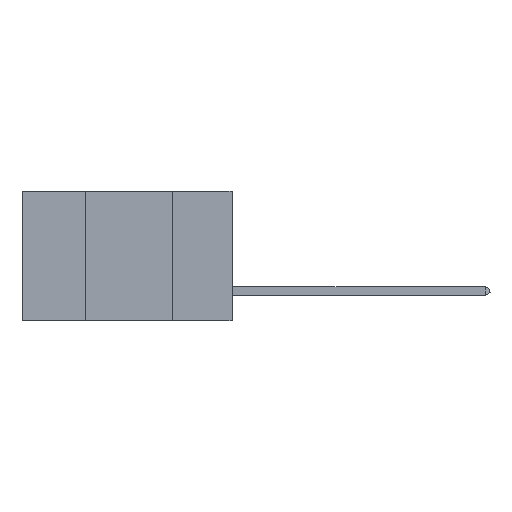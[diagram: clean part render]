
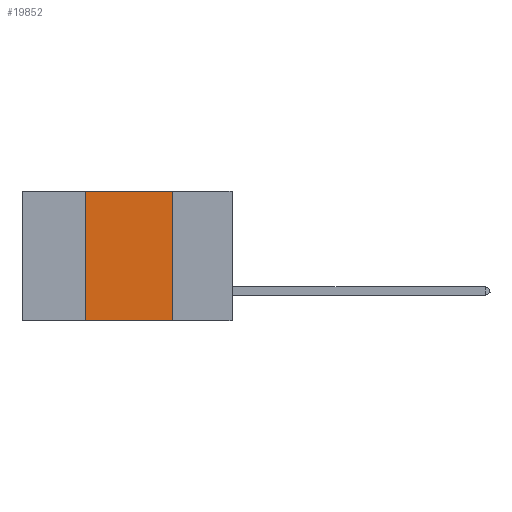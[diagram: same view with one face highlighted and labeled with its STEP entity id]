
A CAD part, left-side view. The second image highlights one B-rep face of the part: STEP entity #19852.
In plain terms, the highlighted planar face has unit normal (-1, 0, 0).
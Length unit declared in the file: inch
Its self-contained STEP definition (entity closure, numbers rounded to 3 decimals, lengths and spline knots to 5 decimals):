
#496 = ORIENTED_EDGE ( 'NONE', *, *, #3935, .F. ) ;
#1645 = CARTESIAN_POINT ( 'NONE',  ( 0., 0.6, 0. ) ) ;
#2488 = CARTESIAN_POINT ( 'NONE',  ( 0., 0.6, -0.37 ) ) ;
#3166 = CARTESIAN_POINT ( 'NONE',  ( 0., 0.42, 0. ) ) ;
#3935 = EDGE_CURVE ( 'NONE', #10370, #10588, #13559, .T. ) ;
#4837 = ORIENTED_EDGE ( 'NONE', *, *, #19130, .F. ) ;
#5339 = CARTESIAN_POINT ( 'NONE',  ( 0., 0.42, -0.37 ) ) ;
#6425 = VECTOR ( 'NONE', #16817, 39.37008 ) ;
#6759 = EDGE_CURVE ( 'NONE', #10370, #9768, #7159, .T. ) ;
#7159 = LINE ( 'NONE', #2488, #6425 ) ;
#7285 = CARTESIAN_POINT ( 'NONE',  ( 0., 0.6, 0. ) ) ;
#9012 = EDGE_CURVE ( 'NONE', #20613, #9768, #12466, .T. ) ;
#9768 = VERTEX_POINT ( 'NONE', #16465 ) ;
#10230 = DIRECTION ( 'NONE',  ( 0., -1., 0. ) ) ;
#10370 = VERTEX_POINT ( 'NONE', #5339 ) ;
#10588 = VERTEX_POINT ( 'NONE', #3166 ) ;
#11583 = DIRECTION ( 'NONE',  ( 1., 0., 0. ) ) ;
#12466 = LINE ( 'NONE', #24455, #23937 ) ;
#13559 = LINE ( 'NONE', #23065, #20819 ) ;
#14512 = DIRECTION ( 'NONE',  ( 0., 0., -1. ) ) ;
#16465 = CARTESIAN_POINT ( 'NONE',  ( 0., 0.17, -0.37 ) ) ;
#16817 = DIRECTION ( 'NONE',  ( 0., -1., 0. ) ) ;
#17622 = DIRECTION ( 'NONE',  ( 0., 0., 1. ) ) ;
#17919 = CARTESIAN_POINT ( 'NONE',  ( 0., 0.17, 0. ) ) ;
#18205 = ORIENTED_EDGE ( 'NONE', *, *, #9012, .F. ) ;
#19130 = EDGE_CURVE ( 'NONE', #10588, #20613, #26587, .T. ) ;
#19852 = ADVANCED_FACE ( 'NONE', ( #23416 ), #20785, .F. ) ;
#20613 = VERTEX_POINT ( 'NONE', #17919 ) ;
#20644 = DIRECTION ( 'NONE',  ( 0., 0., -1. ) ) ;
#20785 = PLANE ( 'NONE',  #27585 ) ;
#20819 = VECTOR ( 'NONE', #17622, 39.37008 ) ;
#20826 = ORIENTED_EDGE ( 'NONE', *, *, #6759, .T. ) ;
#23065 = CARTESIAN_POINT ( 'NONE',  ( 0., 0.42, 0. ) ) ;
#23416 = FACE_OUTER_BOUND ( 'NONE', #26038, .T. ) ;
#23937 = VECTOR ( 'NONE', #14512, 39.37008 ) ;
#24455 = CARTESIAN_POINT ( 'NONE',  ( 0., 0.17, 0. ) ) ;
#26038 = EDGE_LOOP ( 'NONE', ( #18205, #4837, #496, #20826 ) ) ;
#26587 = LINE ( 'NONE', #7285, #29024 ) ;
#27585 = AXIS2_PLACEMENT_3D ( 'NONE', #1645, #11583, #20644 ) ;
#29024 = VECTOR ( 'NONE', #10230, 39.37008 ) ;
